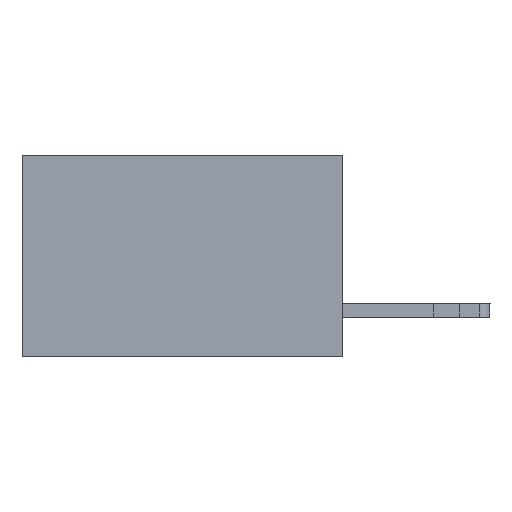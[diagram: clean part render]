
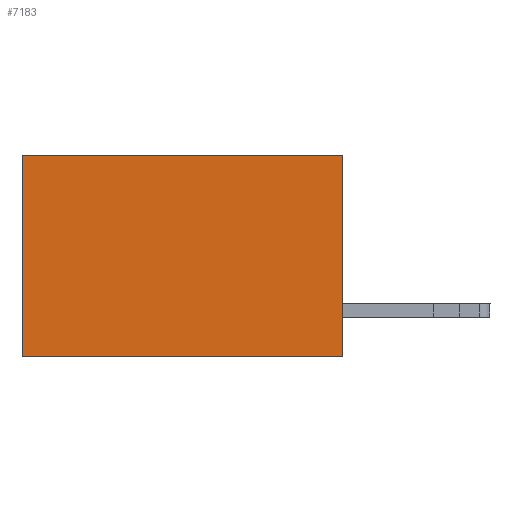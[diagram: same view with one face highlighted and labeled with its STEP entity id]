
A CAD part, left-side view. The second image highlights one B-rep face of the part: STEP entity #7183.
In plain terms, the highlighted planar face has unit normal (-1, 0, 0).
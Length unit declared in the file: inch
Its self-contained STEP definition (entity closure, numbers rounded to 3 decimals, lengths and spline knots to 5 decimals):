
#1462 = LINE ( 'NONE', #7572, #8976 ) ;
#1556 = DIRECTION ( 'NONE',  ( 0., 0., -1. ) ) ;
#4456 = CARTESIAN_POINT ( 'NONE',  ( 0.277, 0.59, -0.37 ) ) ;
#4494 = PLANE ( 'NONE',  #8284 ) ;
#5171 = LINE ( 'NONE', #15926, #12722 ) ;
#5865 = VERTEX_POINT ( 'NONE', #16472 ) ;
#6031 = EDGE_CURVE ( 'NONE', #8699, #8392, #15078, .T. ) ;
#6991 = LINE ( 'NONE', #14588, #10067 ) ;
#7069 = VECTOR ( 'NONE', #13453, 39.37008 ) ;
#7081 = DIRECTION ( 'NONE',  ( 0., 0., -1. ) ) ;
#7183 = ADVANCED_FACE ( 'NONE', ( #9658 ), #4494, .F. ) ;
#7572 = CARTESIAN_POINT ( 'NONE',  ( 0.277, 0., 0. ) ) ;
#8284 = AXIS2_PLACEMENT_3D ( 'NONE', #18067, #10569, #1556 ) ;
#8392 = VERTEX_POINT ( 'NONE', #4456 ) ;
#8699 = VERTEX_POINT ( 'NONE', #9736 ) ;
#8976 = VECTOR ( 'NONE', #10688, 39.37008 ) ;
#9658 = FACE_OUTER_BOUND ( 'NONE', #12802, .T. ) ;
#9715 = VERTEX_POINT ( 'NONE', #16529 ) ;
#9736 = CARTESIAN_POINT ( 'NONE',  ( 0.277, 0., -0.37 ) ) ;
#10067 = VECTOR ( 'NONE', #7081, 39.37008 ) ;
#10569 = DIRECTION ( 'NONE',  ( 1., 0., 0. ) ) ;
#10688 = DIRECTION ( 'NONE',  ( 0., 1., 0. ) ) ;
#11226 = EDGE_CURVE ( 'NONE', #9715, #5865, #1462, .T. ) ;
#12106 = ORIENTED_EDGE ( 'NONE', *, *, #11226, .T. ) ;
#12722 = VECTOR ( 'NONE', #17451, 39.37008 ) ;
#12802 = EDGE_LOOP ( 'NONE', ( #14367, #14351, #16076, #12106 ) ) ;
#13453 = DIRECTION ( 'NONE',  ( 0., 1., 0. ) ) ;
#13554 = EDGE_CURVE ( 'NONE', #5865, #8392, #6991, .T. ) ;
#13754 = CARTESIAN_POINT ( 'NONE',  ( 0.277, 0., -0.37 ) ) ;
#14351 = ORIENTED_EDGE ( 'NONE', *, *, #6031, .F. ) ;
#14367 = ORIENTED_EDGE ( 'NONE', *, *, #13554, .T. ) ;
#14588 = CARTESIAN_POINT ( 'NONE',  ( 0.277, 0.59, -0.37 ) ) ;
#15078 = LINE ( 'NONE', #13754, #7069 ) ;
#15926 = CARTESIAN_POINT ( 'NONE',  ( 0.277, 0., -0.37 ) ) ;
#16076 = ORIENTED_EDGE ( 'NONE', *, *, #17712, .F. ) ;
#16472 = CARTESIAN_POINT ( 'NONE',  ( 0.277, 0.59, 0. ) ) ;
#16529 = CARTESIAN_POINT ( 'NONE',  ( 0.277, 0., 0. ) ) ;
#17451 = DIRECTION ( 'NONE',  ( 0., 0., -1. ) ) ;
#17712 = EDGE_CURVE ( 'NONE', #9715, #8699, #5171, .T. ) ;
#18067 = CARTESIAN_POINT ( 'NONE',  ( 0.277, 0., -0.37 ) ) ;
